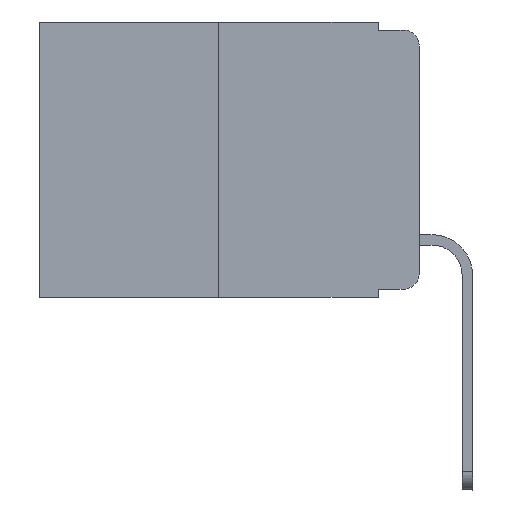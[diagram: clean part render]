
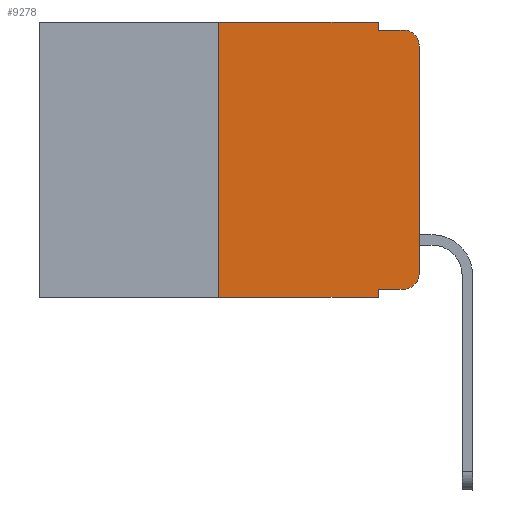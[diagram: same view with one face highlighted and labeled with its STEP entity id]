
A CAD part, left-side view. The second image highlights one B-rep face of the part: STEP entity #9278.
In plain terms, the highlighted planar face has unit normal (-1, 0, 0).
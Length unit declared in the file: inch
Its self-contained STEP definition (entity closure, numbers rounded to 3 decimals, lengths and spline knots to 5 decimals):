
#97 = VERTEX_POINT ( 'NONE', #2854 ) ;
#178 = CARTESIAN_POINT ( 'NONE',  ( 0., 0.25, -0.343 ) ) ;
#232 = VERTEX_POINT ( 'NONE', #11078 ) ;
#265 = CARTESIAN_POINT ( 'NONE',  ( 0., 0.25, 0. ) ) ;
#486 = VERTEX_POINT ( 'NONE', #8077 ) ;
#661 = LINE ( 'NONE', #8783, #2438 ) ;
#768 = VERTEX_POINT ( 'NONE', #11333 ) ;
#1141 = CARTESIAN_POINT ( 'NONE',  ( 0., 0.051, -0.333 ) ) ;
#1616 = EDGE_CURVE ( 'NONE', #768, #8245, #5517, .T. ) ;
#1711 = VECTOR ( 'NONE', #7660, 39.37008 ) ;
#1933 = EDGE_CURVE ( 'NONE', #486, #768, #3021, .T. ) ;
#2390 = CARTESIAN_POINT ( 'NONE',  ( 0., 0.051, -0.01 ) ) ;
#2438 = VECTOR ( 'NONE', #3414, 39.37008 ) ;
#2450 = LINE ( 'NONE', #2390, #6522 ) ;
#2510 = DIRECTION ( 'NONE',  ( 0., -1., 0. ) ) ;
#2540 = AXIS2_PLACEMENT_3D ( 'NONE', #6847, #3318, #7974 ) ;
#2676 = CARTESIAN_POINT ( 'NONE',  ( 0., 0.473, 0. ) ) ;
#2854 = CARTESIAN_POINT ( 'NONE',  ( 0., 0.051, -0.01 ) ) ;
#2959 = EDGE_CURVE ( 'NONE', #4041, #486, #7423, .T. ) ;
#3021 = LINE ( 'NONE', #6489, #9757 ) ;
#3107 = ORIENTED_EDGE ( 'NONE', *, *, #1933, .T. ) ;
#3318 = DIRECTION ( 'NONE',  ( -1., 0., 0. ) ) ;
#3414 = DIRECTION ( 'NONE',  ( 0., -1., 0. ) ) ;
#3495 = PLANE ( 'NONE',  #9792 ) ;
#3635 = DIRECTION ( 'NONE',  ( 0., -1., 0. ) ) ;
#4012 = DIRECTION ( 'NONE',  ( 0., 0., 1. ) ) ;
#4028 = DIRECTION ( 'NONE',  ( -1., 0., 0. ) ) ;
#4041 = VERTEX_POINT ( 'NONE', #7460 ) ;
#4221 = VERTEX_POINT ( 'NONE', #1141 ) ;
#4404 = ORIENTED_EDGE ( 'NONE', *, *, #9510, .T. ) ;
#4726 = EDGE_CURVE ( 'NONE', #9948, #97, #7938, .T. ) ;
#4839 = ORIENTED_EDGE ( 'NONE', *, *, #6049, .T. ) ;
#4855 = DIRECTION ( 'NONE',  ( 0., 0., -1. ) ) ;
#5108 = EDGE_CURVE ( 'NONE', #97, #8245, #2450, .T. ) ;
#5171 = CARTESIAN_POINT ( 'NONE',  ( 0., 0.051, 0. ) ) ;
#5379 = DIRECTION ( 'NONE',  ( 0., 0., -1. ) ) ;
#5517 = CIRCLE ( 'NONE', #10216, 0.02 ) ;
#5605 = LINE ( 'NONE', #6481, #10371 ) ;
#6049 = EDGE_CURVE ( 'NONE', #6949, #8716, #9002, .T. ) ;
#6111 = ORIENTED_EDGE ( 'NONE', *, *, #4726, .F. ) ;
#6441 = ORIENTED_EDGE ( 'NONE', *, *, #11058, .F. ) ;
#6481 = CARTESIAN_POINT ( 'NONE',  ( 0., 0.051, 0. ) ) ;
#6489 = CARTESIAN_POINT ( 'NONE',  ( 0., 0., 0. ) ) ;
#6522 = VECTOR ( 'NONE', #2510, 39.37008 ) ;
#6532 = DIRECTION ( 'NONE',  ( 0., 0., -1. ) ) ;
#6804 = EDGE_LOOP ( 'NONE', ( #3107, #10973, #6826, #6111, #7716, #11074, #4839, #6441, #4404, #9697 ) ) ;
#6826 = ORIENTED_EDGE ( 'NONE', *, *, #5108, .F. ) ;
#6847 = CARTESIAN_POINT ( 'NONE',  ( 0., 0.02, -0.313 ) ) ;
#6949 = VERTEX_POINT ( 'NONE', #178 ) ;
#7302 = EDGE_CURVE ( 'NONE', #232, #9948, #661, .T. ) ;
#7423 = CIRCLE ( 'NONE', #2540, 0.02 ) ;
#7460 = CARTESIAN_POINT ( 'NONE',  ( 0., 0.02, -0.333 ) ) ;
#7552 = CARTESIAN_POINT ( 'NONE',  ( 0., 0.051, -0.333 ) ) ;
#7660 = DIRECTION ( 'NONE',  ( 0., -1., 0. ) ) ;
#7716 = ORIENTED_EDGE ( 'NONE', *, *, #7302, .F. ) ;
#7938 = LINE ( 'NONE', #5171, #11565 ) ;
#7974 = DIRECTION ( 'NONE',  ( 0., 0., -1. ) ) ;
#8077 = CARTESIAN_POINT ( 'NONE',  ( 0., 0., -0.313 ) ) ;
#8245 = VERTEX_POINT ( 'NONE', #9535 ) ;
#8387 = LINE ( 'NONE', #265, #9229 ) ;
#8716 = VERTEX_POINT ( 'NONE', #9463 ) ;
#8783 = CARTESIAN_POINT ( 'NONE',  ( 0., 0.473, 0. ) ) ;
#9002 = LINE ( 'NONE', #10820, #9174 ) ;
#9174 = VECTOR ( 'NONE', #3635, 39.37008 ) ;
#9229 = VECTOR ( 'NONE', #9275, 39.37008 ) ;
#9275 = DIRECTION ( 'NONE',  ( 0., 0., 1. ) ) ;
#9278 = ADVANCED_FACE ( 'NONE', ( #10740 ), #3495, .F. ) ;
#9463 = CARTESIAN_POINT ( 'NONE',  ( 0., 0.051, -0.343 ) ) ;
#9510 = EDGE_CURVE ( 'NONE', #4221, #4041, #11176, .T. ) ;
#9535 = CARTESIAN_POINT ( 'NONE',  ( 0., 0.02, -0.01 ) ) ;
#9697 = ORIENTED_EDGE ( 'NONE', *, *, #2959, .T. ) ;
#9711 = DIRECTION ( 'NONE',  ( 0., 0., -1. ) ) ;
#9757 = VECTOR ( 'NONE', #4012, 39.37008 ) ;
#9792 = AXIS2_PLACEMENT_3D ( 'NONE', #2676, #11474, #5379 ) ;
#9948 = VERTEX_POINT ( 'NONE', #11364 ) ;
#10216 = AXIS2_PLACEMENT_3D ( 'NONE', #10267, #4028, #4855 ) ;
#10267 = CARTESIAN_POINT ( 'NONE',  ( 0., 0.02, -0.03 ) ) ;
#10293 = EDGE_CURVE ( 'NONE', #6949, #232, #8387, .T. ) ;
#10371 = VECTOR ( 'NONE', #6532, 39.37008 ) ;
#10740 = FACE_OUTER_BOUND ( 'NONE', #6804, .T. ) ;
#10820 = CARTESIAN_POINT ( 'NONE',  ( 0., 0.473, -0.343 ) ) ;
#10973 = ORIENTED_EDGE ( 'NONE', *, *, #1616, .T. ) ;
#11058 = EDGE_CURVE ( 'NONE', #4221, #8716, #5605, .T. ) ;
#11074 = ORIENTED_EDGE ( 'NONE', *, *, #10293, .F. ) ;
#11078 = CARTESIAN_POINT ( 'NONE',  ( 0., 0.25, 0. ) ) ;
#11176 = LINE ( 'NONE', #7552, #1711 ) ;
#11333 = CARTESIAN_POINT ( 'NONE',  ( 0., 0., -0.03 ) ) ;
#11364 = CARTESIAN_POINT ( 'NONE',  ( 0., 0.051, 0. ) ) ;
#11474 = DIRECTION ( 'NONE',  ( 1., 0., 0. ) ) ;
#11565 = VECTOR ( 'NONE', #9711, 39.37008 ) ;
